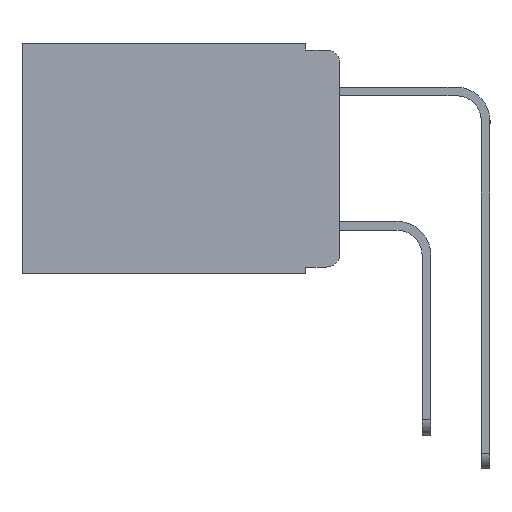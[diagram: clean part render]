
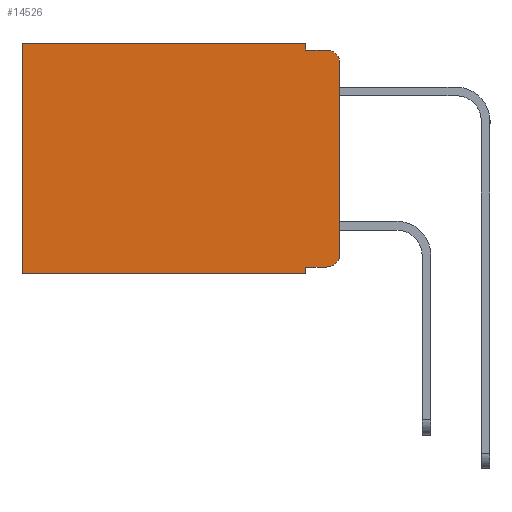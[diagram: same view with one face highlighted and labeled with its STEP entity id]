
A CAD part, left-side view. The second image highlights one B-rep face of the part: STEP entity #14526.
In plain terms, the highlighted planar face has unit normal (-1, 0, 0).
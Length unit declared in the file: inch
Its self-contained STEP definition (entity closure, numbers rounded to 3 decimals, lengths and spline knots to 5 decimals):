
#35 = CARTESIAN_POINT ( 'NONE',  ( 0.298, 0.051, -0.343 ) ) ;
#94 = ORIENTED_EDGE ( 'NONE', *, *, #8934, .F. ) ;
#276 = DIRECTION ( 'NONE',  ( 0., 0., -1. ) ) ;
#559 = CARTESIAN_POINT ( 'NONE',  ( 0.298, 0.02, -0.01 ) ) ;
#785 = DIRECTION ( 'NONE',  ( -1., 0., 0. ) ) ;
#797 = LINE ( 'NONE', #8093, #8609 ) ;
#1107 = DIRECTION ( 'NONE',  ( -1., 0., 0. ) ) ;
#1174 = VERTEX_POINT ( 'NONE', #15191 ) ;
#1195 = CARTESIAN_POINT ( 'NONE',  ( 0.298, 0., 0. ) ) ;
#1381 = EDGE_CURVE ( 'NONE', #8693, #4121, #13737, .T. ) ;
#1576 = ORIENTED_EDGE ( 'NONE', *, *, #6653, .T. ) ;
#1597 = ORIENTED_EDGE ( 'NONE', *, *, #9436, .T. ) ;
#1730 = CARTESIAN_POINT ( 'NONE',  ( 0.298, 0., 0. ) ) ;
#1971 = ORIENTED_EDGE ( 'NONE', *, *, #6096, .F. ) ;
#3408 = CARTESIAN_POINT ( 'NONE',  ( 0.298, 0., -0.313 ) ) ;
#3419 = ORIENTED_EDGE ( 'NONE', *, *, #1381, .F. ) ;
#3517 = CARTESIAN_POINT ( 'NONE',  ( 0.298, 0., -0.03 ) ) ;
#3800 = ORIENTED_EDGE ( 'NONE', *, *, #12940, .T. ) ;
#4121 = VERTEX_POINT ( 'NONE', #3408 ) ;
#4950 = VECTOR ( 'NONE', #7962, 39.37008 ) ;
#5054 = EDGE_CURVE ( 'NONE', #11883, #11815, #12760, .T. ) ;
#5150 = LINE ( 'NONE', #14592, #8713 ) ;
#5252 = VECTOR ( 'NONE', #15151, 39.37008 ) ;
#5540 = AXIS2_PLACEMENT_3D ( 'NONE', #10325, #1107, #11737 ) ;
#5691 = CARTESIAN_POINT ( 'NONE',  ( 0.298, 0.051, -0.01 ) ) ;
#5738 = LINE ( 'NONE', #1730, #5252 ) ;
#5776 = DIRECTION ( 'NONE',  ( 0., 1., 0. ) ) ;
#6091 = AXIS2_PLACEMENT_3D ( 'NONE', #10038, #785, #11451 ) ;
#6096 = EDGE_CURVE ( 'NONE', #11815, #10246, #18364, .T. ) ;
#6499 = VECTOR ( 'NONE', #7113, 39.37008 ) ;
#6653 = EDGE_CURVE ( 'NONE', #8693, #10246, #8672, .T. ) ;
#6932 = VECTOR ( 'NONE', #5776, 39.37008 ) ;
#7041 = CARTESIAN_POINT ( 'NONE',  ( 0.298, 0., 0. ) ) ;
#7113 = DIRECTION ( 'NONE',  ( 0., 0., -1. ) ) ;
#7501 = DIRECTION ( 'NONE',  ( 0., 0., -1. ) ) ;
#7692 = AXIS2_PLACEMENT_3D ( 'NONE', #1195, #16050, #7501 ) ;
#7962 = DIRECTION ( 'NONE',  ( 0., 0., -1. ) ) ;
#8093 = CARTESIAN_POINT ( 'NONE',  ( 0.298, 0.473, 0. ) ) ;
#8160 = ORIENTED_EDGE ( 'NONE', *, *, #5054, .F. ) ;
#8267 = CARTESIAN_POINT ( 'NONE',  ( 0.298, 0.051, 0. ) ) ;
#8609 = VECTOR ( 'NONE', #276, 39.37008 ) ;
#8672 = CIRCLE ( 'NONE', #6091, 0.02 ) ;
#8683 = EDGE_CURVE ( 'NONE', #15426, #1174, #797, .T. ) ;
#8693 = VERTEX_POINT ( 'NONE', #3517 ) ;
#8713 = VECTOR ( 'NONE', #15991, 39.37008 ) ;
#8934 = EDGE_CURVE ( 'NONE', #17120, #1174, #18275, .T. ) ;
#9436 = EDGE_CURVE ( 'NONE', #11883, #15426, #5738, .T. ) ;
#9876 = CARTESIAN_POINT ( 'NONE',  ( 0.298, 0.051, 0. ) ) ;
#10038 = CARTESIAN_POINT ( 'NONE',  ( 0.298, 0.02, -0.03 ) ) ;
#10147 = ORIENTED_EDGE ( 'NONE', *, *, #11986, .T. ) ;
#10246 = VERTEX_POINT ( 'NONE', #559 ) ;
#10325 = CARTESIAN_POINT ( 'NONE',  ( 0.298, 0.02, -0.313 ) ) ;
#10768 = VERTEX_POINT ( 'NONE', #12153 ) ;
#11011 = EDGE_CURVE ( 'NONE', #10768, #17120, #19043, .T. ) ;
#11156 = FACE_OUTER_BOUND ( 'NONE', #17824, .T. ) ;
#11273 = ORIENTED_EDGE ( 'NONE', *, *, #11011, .F. ) ;
#11451 = DIRECTION ( 'NONE',  ( 0., 0., -1. ) ) ;
#11522 = ORIENTED_EDGE ( 'NONE', *, *, #8683, .T. ) ;
#11643 = VECTOR ( 'NONE', #16728, 39.37008 ) ;
#11737 = DIRECTION ( 'NONE',  ( 0., 0., -1. ) ) ;
#11815 = VERTEX_POINT ( 'NONE', #16652 ) ;
#11883 = VERTEX_POINT ( 'NONE', #15502 ) ;
#11986 = EDGE_CURVE ( 'NONE', #10768, #12092, #5150, .T. ) ;
#12092 = VERTEX_POINT ( 'NONE', #14777 ) ;
#12153 = CARTESIAN_POINT ( 'NONE',  ( 0.298, 0.051, -0.333 ) ) ;
#12760 = LINE ( 'NONE', #9876, #4950 ) ;
#12940 = EDGE_CURVE ( 'NONE', #12092, #4121, #14675, .T. ) ;
#13028 = CARTESIAN_POINT ( 'NONE',  ( 0.298, 0., -0.343 ) ) ;
#13737 = LINE ( 'NONE', #7041, #6499 ) ;
#14526 = ADVANCED_FACE ( 'NONE', ( #11156 ), #14660, .F. ) ;
#14592 = CARTESIAN_POINT ( 'NONE',  ( 0.298, 0.051, -0.333 ) ) ;
#14660 = PLANE ( 'NONE',  #7692 ) ;
#14675 = CIRCLE ( 'NONE', #5540, 0.02 ) ;
#14777 = CARTESIAN_POINT ( 'NONE',  ( 0.298, 0.02, -0.333 ) ) ;
#15151 = DIRECTION ( 'NONE',  ( 0., 1., 0. ) ) ;
#15191 = CARTESIAN_POINT ( 'NONE',  ( 0.298, 0.473, -0.343 ) ) ;
#15426 = VERTEX_POINT ( 'NONE', #16318 ) ;
#15502 = CARTESIAN_POINT ( 'NONE',  ( 0.298, 0.051, 0. ) ) ;
#15632 = DIRECTION ( 'NONE',  ( 0., -1., 0. ) ) ;
#15991 = DIRECTION ( 'NONE',  ( 0., -1., 0. ) ) ;
#16050 = DIRECTION ( 'NONE',  ( 1., 0., 0. ) ) ;
#16318 = CARTESIAN_POINT ( 'NONE',  ( 0.298, 0.473, 0. ) ) ;
#16652 = CARTESIAN_POINT ( 'NONE',  ( 0.298, 0.051, -0.01 ) ) ;
#16728 = DIRECTION ( 'NONE',  ( 0., 0., -1. ) ) ;
#17120 = VERTEX_POINT ( 'NONE', #35 ) ;
#17824 = EDGE_LOOP ( 'NONE', ( #3419, #1576, #1971, #8160, #1597, #11522, #94, #11273, #10147, #3800 ) ) ;
#17929 = VECTOR ( 'NONE', #15632, 39.37008 ) ;
#18275 = LINE ( 'NONE', #13028, #6932 ) ;
#18364 = LINE ( 'NONE', #5691, #17929 ) ;
#19043 = LINE ( 'NONE', #8267, #11643 ) ;
